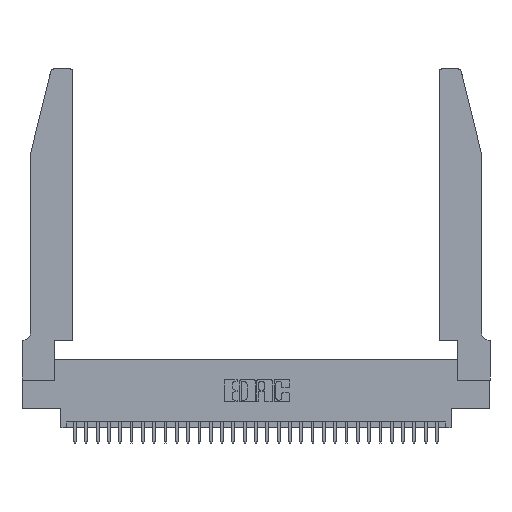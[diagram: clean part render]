
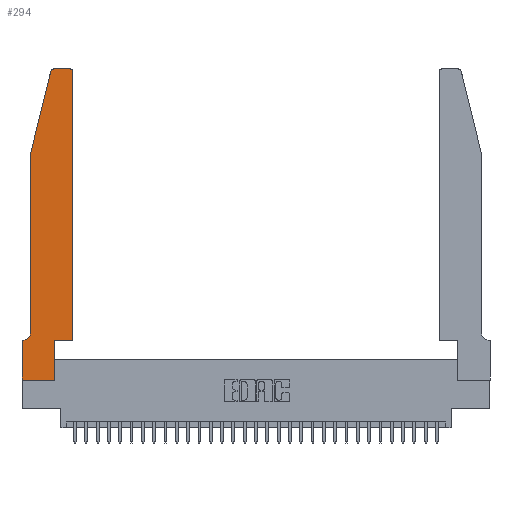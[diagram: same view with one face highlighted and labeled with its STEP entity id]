
A CAD part, top view. The second image highlights one B-rep face of the part: STEP entity #294.
In plain terms, the highlighted planar face has unit normal (0, 0, 1).
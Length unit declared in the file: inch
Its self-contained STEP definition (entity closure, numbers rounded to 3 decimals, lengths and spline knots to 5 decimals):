
#147 = VERTEX_POINT ( 'NONE', #22132 ) ;
#294 = ADVANCED_FACE ( 'NONE', ( #4234 ), #27703, .T. ) ;
#302 = VECTOR ( 'NONE', #12149, 39.37008 ) ;
#444 = DIRECTION ( 'NONE',  ( 1., 0., 0. ) ) ;
#767 = ORIENTED_EDGE ( 'NONE', *, *, #31641, .T. ) ;
#1257 = ORIENTED_EDGE ( 'NONE', *, *, #4032, .T. ) ;
#1688 = CARTESIAN_POINT ( 'NONE',  ( 0.2865, 0.35, 0.37 ) ) ;
#1886 = EDGE_CURVE ( 'NONE', #14572, #8402, #8769, .T. ) ;
#2227 = VERTEX_POINT ( 'NONE', #4747 ) ;
#2952 = CIRCLE ( 'NONE', #5189, 0.03 ) ;
#3463 = VERTEX_POINT ( 'NONE', #11532 ) ;
#3545 = DIRECTION ( 'NONE',  ( 1., 0., 0. ) ) ;
#3991 = ORIENTED_EDGE ( 'NONE', *, *, #26166, .T. ) ;
#4032 = EDGE_CURVE ( 'NONE', #2227, #25944, #26234, .T. ) ;
#4234 = FACE_OUTER_BOUND ( 'NONE', #17159, .T. ) ;
#4522 = EDGE_CURVE ( 'NONE', #25625, #2227, #30083, .T. ) ;
#4747 = CARTESIAN_POINT ( 'NONE',  ( 0.2865, 0., 0.37 ) ) ;
#5189 = AXIS2_PLACEMENT_3D ( 'NONE', #18276, #30212, #28162 ) ;
#5870 = VERTEX_POINT ( 'NONE', #6015 ) ;
#5938 = EDGE_CURVE ( 'NONE', #8402, #8376, #22321, .T. ) ;
#5988 = VERTEX_POINT ( 'NONE', #24692 ) ;
#6015 = CARTESIAN_POINT ( 'NONE',  ( 0.0055, 0.35, 0.37 ) ) ;
#6142 = EDGE_CURVE ( 'NONE', #3463, #23357, #7967, .T. ) ;
#6798 = CIRCLE ( 'NONE', #22216, 0.07 ) ;
#7615 = DIRECTION ( 'NONE',  ( -0.239, -0.971, 0. ) ) ;
#7659 = VECTOR ( 'NONE', #444, 39.37008 ) ;
#7678 = DIRECTION ( 'NONE',  ( -1., 0., 0. ) ) ;
#7967 = LINE ( 'NONE', #16505, #8748 ) ;
#8073 = DIRECTION ( 'NONE',  ( 0., 0., 1. ) ) ;
#8367 = DIRECTION ( 'NONE',  ( 1., 0., 0. ) ) ;
#8376 = VERTEX_POINT ( 'NONE', #8736 ) ;
#8402 = VERTEX_POINT ( 'NONE', #29588 ) ;
#8600 = ORIENTED_EDGE ( 'NONE', *, *, #4522, .T. ) ;
#8736 = CARTESIAN_POINT ( 'NONE',  ( 0.25487, 2.72718, 0.37 ) ) ;
#8748 = VECTOR ( 'NONE', #28766, 39.37008 ) ;
#8769 = LINE ( 'NONE', #20127, #23880 ) ;
#9922 = EDGE_CURVE ( 'NONE', #147, #25625, #16986, .T. ) ;
#10049 = CARTESIAN_POINT ( 'NONE',  ( 0., 0., 0.37 ) ) ;
#10338 = CARTESIAN_POINT ( 'NONE',  ( 0., 0.35, 0.37 ) ) ;
#10704 = CARTESIAN_POINT ( 'NONE',  ( 0., 0., 0.37 ) ) ;
#10938 = ORIENTED_EDGE ( 'NONE', *, *, #6142, .T. ) ;
#10986 = LINE ( 'NONE', #31099, #12553 ) ;
#11116 = ORIENTED_EDGE ( 'NONE', *, *, #28636, .T. ) ;
#11532 = CARTESIAN_POINT ( 'NONE',  ( 0.0755, 2., 0.37 ) ) ;
#11967 = VECTOR ( 'NONE', #21057, 39.37008 ) ;
#12149 = DIRECTION ( 'NONE',  ( 0., 1., 0. ) ) ;
#12553 = VECTOR ( 'NONE', #28386, 39.37008 ) ;
#13271 = DIRECTION ( 'NONE',  ( 0., 0., -1. ) ) ;
#13454 = ORIENTED_EDGE ( 'NONE', *, *, #22920, .T. ) ;
#13931 = CARTESIAN_POINT ( 'NONE',  ( 0.4505, 0.35, 0.37 ) ) ;
#14572 = VERTEX_POINT ( 'NONE', #19630 ) ;
#16505 = CARTESIAN_POINT ( 'NONE',  ( 0.0755, 2., 0.37 ) ) ;
#16864 = VECTOR ( 'NONE', #8367, 39.37008 ) ;
#16929 = VERTEX_POINT ( 'NONE', #13931 ) ;
#16986 = LINE ( 'NONE', #21160, #11967 ) ;
#17159 = EDGE_LOOP ( 'NONE', ( #22047, #30754, #11116, #10938, #27397, #13454, #31241, #8600, #1257, #767, #18204, #3991 ) ) ;
#18204 = ORIENTED_EDGE ( 'NONE', *, *, #28936, .T. ) ;
#18276 = CARTESIAN_POINT ( 'NONE',  ( 0.4205, 2.72, 0.37 ) ) ;
#19630 = CARTESIAN_POINT ( 'NONE',  ( 0.4205, 2.75, 0.37 ) ) ;
#20127 = CARTESIAN_POINT ( 'NONE',  ( 0.2605, 2.75, 0.37 ) ) ;
#20174 = CARTESIAN_POINT ( 'NONE',  ( 0.0755, 2., 0.37 ) ) ;
#20912 = DIRECTION ( 'NONE',  ( -1., 0., 0. ) ) ;
#21045 = CARTESIAN_POINT ( 'NONE',  ( 0.0755, 0.35, 0.37 ) ) ;
#21057 = DIRECTION ( 'NONE',  ( 0., -1., 0. ) ) ;
#21160 = CARTESIAN_POINT ( 'NONE',  ( 0., 0., 0.37 ) ) ;
#21533 = VECTOR ( 'NONE', #26417, 39.37008 ) ;
#21937 = CARTESIAN_POINT ( 'NONE',  ( 0.2865, 0.35, 0.37 ) ) ;
#22047 = ORIENTED_EDGE ( 'NONE', *, *, #1886, .T. ) ;
#22132 = CARTESIAN_POINT ( 'NONE',  ( 0., 0.35, 0.37 ) ) ;
#22216 = AXIS2_PLACEMENT_3D ( 'NONE', #28009, #13271, #20912 ) ;
#22321 = CIRCLE ( 'NONE', #26266, 0.03 ) ;
#22920 = EDGE_CURVE ( 'NONE', #5870, #147, #29640, .T. ) ;
#23291 = CARTESIAN_POINT ( 'NONE',  ( 0.4505, 0.35, 0.37 ) ) ;
#23357 = VERTEX_POINT ( 'NONE', #29948 ) ;
#23880 = VECTOR ( 'NONE', #7678, 39.37008 ) ;
#24692 = CARTESIAN_POINT ( 'NONE',  ( 0.4505, 2.72, 0.37 ) ) ;
#25561 = CARTESIAN_POINT ( 'NONE',  ( 0.284, 2.72, 0.37 ) ) ;
#25625 = VERTEX_POINT ( 'NONE', #10704 ) ;
#25944 = VERTEX_POINT ( 'NONE', #1688 ) ;
#26076 = LINE ( 'NONE', #23291, #16864 ) ;
#26166 = EDGE_CURVE ( 'NONE', #5988, #14572, #2952, .T. ) ;
#26234 = LINE ( 'NONE', #21937, #302 ) ;
#26266 = AXIS2_PLACEMENT_3D ( 'NONE', #25561, #8073, #3545 ) ;
#26417 = DIRECTION ( 'NONE',  ( -1., 0., 0. ) ) ;
#26872 = EDGE_CURVE ( 'NONE', #23357, #5870, #6798, .T. ) ;
#27197 = LINE ( 'NONE', #20174, #29925 ) ;
#27397 = ORIENTED_EDGE ( 'NONE', *, *, #26872, .T. ) ;
#27481 = DIRECTION ( 'NONE',  ( 0., 0., 1. ) ) ;
#27703 = PLANE ( 'NONE',  #27716 ) ;
#27716 = AXIS2_PLACEMENT_3D ( 'NONE', #10338, #27481, #30097 ) ;
#28009 = CARTESIAN_POINT ( 'NONE',  ( 0.0055, 0.42, 0.37 ) ) ;
#28162 = DIRECTION ( 'NONE',  ( 1., 0., 0. ) ) ;
#28386 = DIRECTION ( 'NONE',  ( 0., 1., 0. ) ) ;
#28636 = EDGE_CURVE ( 'NONE', #8376, #3463, #27197, .T. ) ;
#28766 = DIRECTION ( 'NONE',  ( 0., -1., 0. ) ) ;
#28936 = EDGE_CURVE ( 'NONE', #16929, #5988, #10986, .T. ) ;
#29588 = CARTESIAN_POINT ( 'NONE',  ( 0.284, 2.75, 0.37 ) ) ;
#29640 = LINE ( 'NONE', #21045, #21533 ) ;
#29925 = VECTOR ( 'NONE', #7615, 39.37008 ) ;
#29948 = CARTESIAN_POINT ( 'NONE',  ( 0.0755, 0.42, 0.37 ) ) ;
#30083 = LINE ( 'NONE', #10049, #7659 ) ;
#30097 = DIRECTION ( 'NONE',  ( 1., 0., 0. ) ) ;
#30212 = DIRECTION ( 'NONE',  ( 0., 0., 1. ) ) ;
#30754 = ORIENTED_EDGE ( 'NONE', *, *, #5938, .T. ) ;
#31099 = CARTESIAN_POINT ( 'NONE',  ( 0.4505, 0.35, 0.37 ) ) ;
#31241 = ORIENTED_EDGE ( 'NONE', *, *, #9922, .T. ) ;
#31641 = EDGE_CURVE ( 'NONE', #25944, #16929, #26076, .T. ) ;
